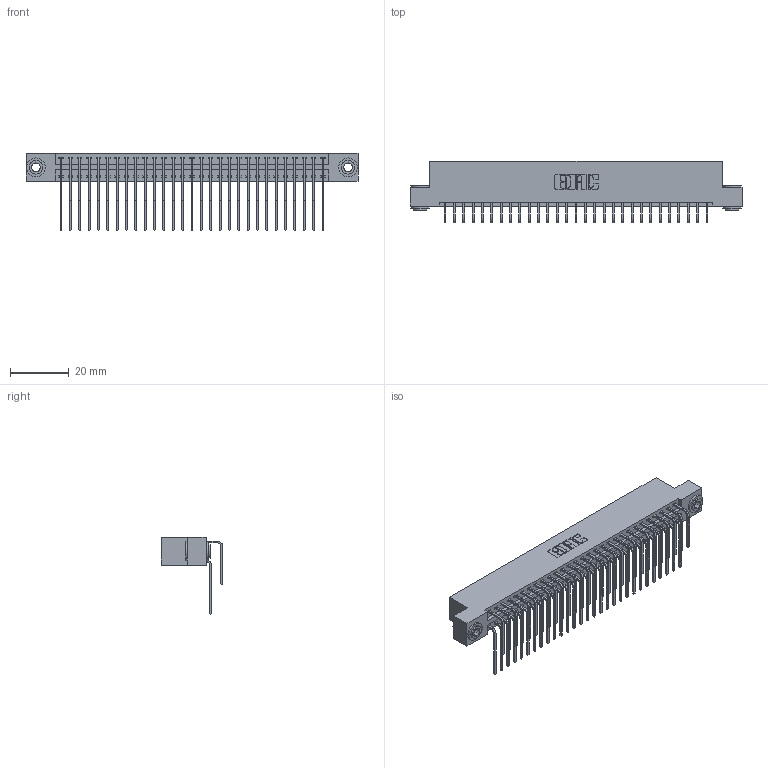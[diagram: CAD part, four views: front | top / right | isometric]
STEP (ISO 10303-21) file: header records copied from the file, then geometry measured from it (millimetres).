
FILE_DESCRIPTION (( 'STEP AP203' ), '1' );
FILE_NAME ('346-058-559-203.STEP', '2022-05-21T09:35:11', ( '' ), ( '' ), 'SwSTEP 2.0', 'SolidWorks 2020', '' );
FILE_SCHEMA (( 'CONFIG_CONTROL_DESIGN' ));
Length unit declared in the file: inch
Products named in the file (5): 346-058-559-203; 345-250-002_345-250-002-102; 345-292-001_559 Tail - 2; 345-292-001_558 559 Tail - 1; 346 Part_Flush Mounting Lugs - 0.156 Dia-TH
Assembly tree (61 placements, depth 2):
  346-058-559-203
    346 Part_Flush Mounting Lugs - 0.156 Dia-TH
    345-292-001_558 559 Tail - 1  x29
    345-292-001_559 Tail - 2  x29
    345-250-002_345-250-002-102  x2
Bounding box: 112.65 x 20.89 x 26.16 mm (x, y, z)
Volume: 11219.6 mm3; surface area: 17071.6 mm2
Topology: 61 solids, 61 shells, 3306 faces, 9779 edges, 6438 vertices
Faces by surface type: plane 2246, cylinder 1052, cone 8
Entity records: 23526 total; most frequent: CARTESIAN_POINT 3928, ORIENTED_EDGE 3802, DIRECTION 3515, EDGE_CURVE 1901, LINE 1589, VECTOR 1589, VERTEX_POINT 1262, AXIS2_PLACEMENT_3D 963
